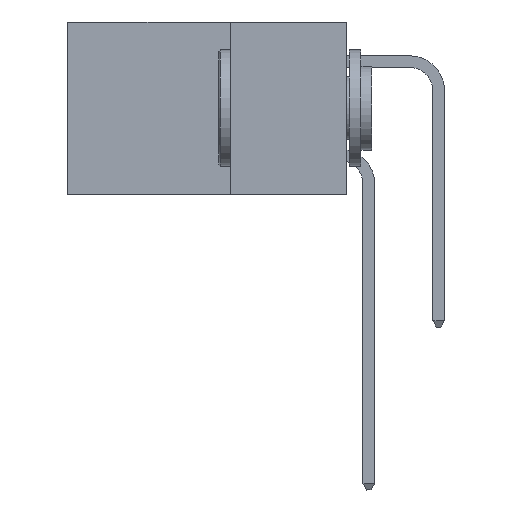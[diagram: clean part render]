
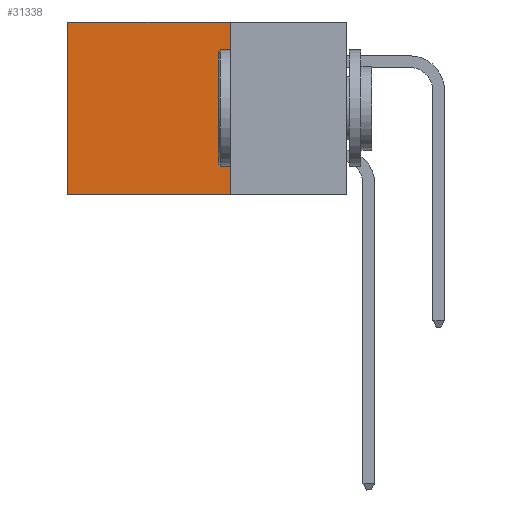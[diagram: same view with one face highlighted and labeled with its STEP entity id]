
A CAD part, left-side view. The second image highlights one B-rep face of the part: STEP entity #31338.
In plain terms, the highlighted planar face has unit normal (-1, 0, 0).
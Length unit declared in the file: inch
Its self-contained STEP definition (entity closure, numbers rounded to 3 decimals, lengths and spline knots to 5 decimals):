
#626 = CARTESIAN_POINT ( 'NONE',  ( 0.2875, 0.6, 0. ) ) ;
#2583 = VERTEX_POINT ( 'NONE', #21687 ) ;
#6047 = CARTESIAN_POINT ( 'NONE',  ( 0.2875, 0.6, -0.37 ) ) ;
#6782 = DIRECTION ( 'NONE',  ( 0., 0., -1. ) ) ;
#6808 = EDGE_CURVE ( 'NONE', #14571, #39144, #28278, .T. ) ;
#8313 = LINE ( 'NONE', #13124, #32551 ) ;
#9291 = ORIENTED_EDGE ( 'NONE', *, *, #26897, .F. ) ;
#9295 = CARTESIAN_POINT ( 'NONE',  ( 0.2875, 0.25, -0.37 ) ) ;
#9883 = CARTESIAN_POINT ( 'NONE',  ( 0.2875, 0.25, 0. ) ) ;
#12745 = VERTEX_POINT ( 'NONE', #16927 ) ;
#13040 = PLANE ( 'NONE',  #33426 ) ;
#13124 = CARTESIAN_POINT ( 'NONE',  ( 0.2875, 0.25, 0. ) ) ;
#14571 = VERTEX_POINT ( 'NONE', #24600 ) ;
#15364 = DIRECTION ( 'NONE',  ( 0., 1., 0. ) ) ;
#16927 = CARTESIAN_POINT ( 'NONE',  ( 0.2875, 0.25, 0. ) ) ;
#19564 = ORIENTED_EDGE ( 'NONE', *, *, #32052, .F. ) ;
#21501 = ORIENTED_EDGE ( 'NONE', *, *, #6808, .T. ) ;
#21687 = CARTESIAN_POINT ( 'NONE',  ( 0.2875, 0.25, -0.37 ) ) ;
#21892 = FACE_OUTER_BOUND ( 'NONE', #26934, .T. ) ;
#22875 = CARTESIAN_POINT ( 'NONE',  ( 0.2875, 0.25, 0. ) ) ;
#23098 = DIRECTION ( 'NONE',  ( 0., 1., 0. ) ) ;
#23143 = DIRECTION ( 'NONE',  ( 1., 0., 0. ) ) ;
#23444 = VECTOR ( 'NONE', #6782, 39.37008 ) ;
#24600 = CARTESIAN_POINT ( 'NONE',  ( 0.2875, 0.6, 0. ) ) ;
#26897 = EDGE_CURVE ( 'NONE', #2583, #39144, #27689, .T. ) ;
#26934 = EDGE_LOOP ( 'NONE', ( #21501, #9291, #19564, #30502 ) ) ;
#27689 = LINE ( 'NONE', #9295, #31278 ) ;
#28278 = LINE ( 'NONE', #626, #28778 ) ;
#28778 = VECTOR ( 'NONE', #39156, 39.37008 ) ;
#30502 = ORIENTED_EDGE ( 'NONE', *, *, #32149, .T. ) ;
#31278 = VECTOR ( 'NONE', #15364, 39.37008 ) ;
#31338 = ADVANCED_FACE ( 'NONE', ( #21892 ), #13040, .F. ) ;
#32052 = EDGE_CURVE ( 'NONE', #12745, #2583, #38095, .T. ) ;
#32149 = EDGE_CURVE ( 'NONE', #12745, #14571, #8313, .T. ) ;
#32551 = VECTOR ( 'NONE', #23098, 39.37008 ) ;
#33426 = AXIS2_PLACEMENT_3D ( 'NONE', #22875, #23143, #39140 ) ;
#38095 = LINE ( 'NONE', #9883, #23444 ) ;
#39140 = DIRECTION ( 'NONE',  ( 0., 0., -1. ) ) ;
#39144 = VERTEX_POINT ( 'NONE', #6047 ) ;
#39156 = DIRECTION ( 'NONE',  ( 0., 0., -1. ) ) ;
